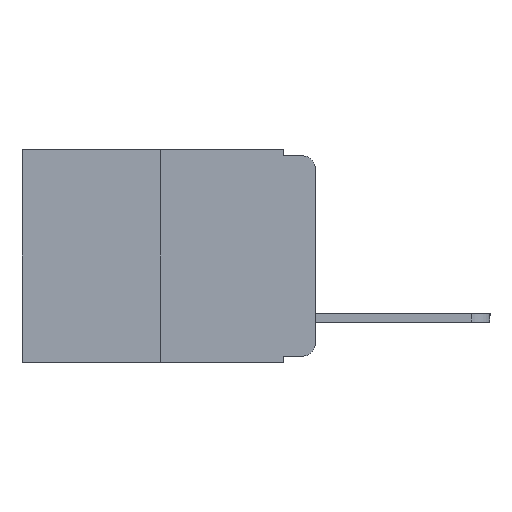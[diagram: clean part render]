
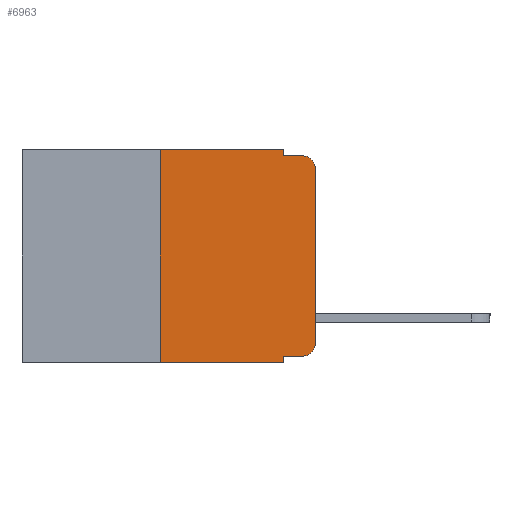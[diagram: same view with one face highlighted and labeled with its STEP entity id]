
A CAD part, left-side view. The second image highlights one B-rep face of the part: STEP entity #6963.
In plain terms, the highlighted planar face has unit normal (-1, 0, 0).
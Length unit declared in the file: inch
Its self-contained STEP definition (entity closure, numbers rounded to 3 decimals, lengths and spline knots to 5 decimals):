
#911 = EDGE_LOOP ( 'NONE', ( #9124, #13321, #1147, #14265, #2266, #7327, #11644, #19059, #3813, #5379 ) ) ;
#1113 = CARTESIAN_POINT ( 'NONE',  ( 0., 0.25, 0. ) ) ;
#1147 = ORIENTED_EDGE ( 'NONE', *, *, #12246, .F. ) ;
#1267 = VECTOR ( 'NONE', #9190, 39.37008 ) ;
#1450 = PLANE ( 'NONE',  #16482 ) ;
#1509 = LINE ( 'NONE', #15160, #9963 ) ;
#1570 = LINE ( 'NONE', #17102, #10512 ) ;
#1821 = LINE ( 'NONE', #10811, #1267 ) ;
#1976 = DIRECTION ( 'NONE',  ( 0., -1., 0. ) ) ;
#2266 = ORIENTED_EDGE ( 'NONE', *, *, #6597, .F. ) ;
#2434 = VERTEX_POINT ( 'NONE', #3434 ) ;
#2712 = EDGE_CURVE ( 'NONE', #18572, #6453, #1509, .T. ) ;
#2749 = VERTEX_POINT ( 'NONE', #3488 ) ;
#3434 = CARTESIAN_POINT ( 'NONE',  ( 0., 0.051, 0. ) ) ;
#3452 = CARTESIAN_POINT ( 'NONE',  ( 0., 0.02, -0.03 ) ) ;
#3488 = CARTESIAN_POINT ( 'NONE',  ( 0., 0.051, -0.333 ) ) ;
#3782 = CARTESIAN_POINT ( 'NONE',  ( 0., 0., 0. ) ) ;
#3813 = ORIENTED_EDGE ( 'NONE', *, *, #15939, .T. ) ;
#3891 = VECTOR ( 'NONE', #7040, 39.37008 ) ;
#3948 = CIRCLE ( 'NONE', #7105, 0.02 ) ;
#4515 = VERTEX_POINT ( 'NONE', #17862 ) ;
#4842 = DIRECTION ( 'NONE',  ( 0., 0., 1. ) ) ;
#5079 = DIRECTION ( 'NONE',  ( 0., 0., -1. ) ) ;
#5379 = ORIENTED_EDGE ( 'NONE', *, *, #11825, .T. ) ;
#5428 = VERTEX_POINT ( 'NONE', #12274 ) ;
#5449 = DIRECTION ( 'NONE',  ( 0., 0., 1. ) ) ;
#5590 = EDGE_CURVE ( 'NONE', #2434, #11676, #1570, .T. ) ;
#5678 = CARTESIAN_POINT ( 'NONE',  ( 0., 0.051, 0. ) ) ;
#5838 = DIRECTION ( 'NONE',  ( -1., 0., 0. ) ) ;
#6208 = VERTEX_POINT ( 'NONE', #19092 ) ;
#6453 = VERTEX_POINT ( 'NONE', #15829 ) ;
#6570 = CARTESIAN_POINT ( 'NONE',  ( 0., 0.051, -0.333 ) ) ;
#6597 = EDGE_CURVE ( 'NONE', #18201, #2434, #8452, .T. ) ;
#6631 = VERTEX_POINT ( 'NONE', #13455 ) ;
#6963 = ADVANCED_FACE ( 'NONE', ( #17617 ), #1450, .F. ) ;
#7040 = DIRECTION ( 'NONE',  ( 0., -1., 0. ) ) ;
#7105 = AXIS2_PLACEMENT_3D ( 'NONE', #15304, #5838, #16618 ) ;
#7327 = ORIENTED_EDGE ( 'NONE', *, *, #16709, .F. ) ;
#7417 = VECTOR ( 'NONE', #5449, 39.37008 ) ;
#8452 = LINE ( 'NONE', #16167, #3891 ) ;
#9124 = ORIENTED_EDGE ( 'NONE', *, *, #18750, .T. ) ;
#9190 = DIRECTION ( 'NONE',  ( 0., -1., 0. ) ) ;
#9215 = VECTOR ( 'NONE', #4842, 39.37008 ) ;
#9225 = LINE ( 'NONE', #5678, #16617 ) ;
#9953 = DIRECTION ( 'NONE',  ( 0., 0., -1. ) ) ;
#9963 = VECTOR ( 'NONE', #1976, 39.37008 ) ;
#10512 = VECTOR ( 'NONE', #17773, 39.37008 ) ;
#10747 = CIRCLE ( 'NONE', #11778, 0.02 ) ;
#10811 = CARTESIAN_POINT ( 'NONE',  ( 0., 0.051, -0.01 ) ) ;
#11644 = ORIENTED_EDGE ( 'NONE', *, *, #2712, .T. ) ;
#11676 = VERTEX_POINT ( 'NONE', #16132 ) ;
#11778 = AXIS2_PLACEMENT_3D ( 'NONE', #3452, #14719, #5079 ) ;
#11825 = EDGE_CURVE ( 'NONE', #5428, #6631, #3948, .T. ) ;
#12236 = LINE ( 'NONE', #6570, #19155 ) ;
#12246 = EDGE_CURVE ( 'NONE', #11676, #6208, #1821, .T. ) ;
#12274 = CARTESIAN_POINT ( 'NONE',  ( 0., 0.02, -0.333 ) ) ;
#13050 = CARTESIAN_POINT ( 'NONE',  ( 0., 0.25, 0. ) ) ;
#13071 = DIRECTION ( 'NONE',  ( 0., -1., 0. ) ) ;
#13321 = ORIENTED_EDGE ( 'NONE', *, *, #16077, .T. ) ;
#13455 = CARTESIAN_POINT ( 'NONE',  ( 0., 0., -0.313 ) ) ;
#14265 = ORIENTED_EDGE ( 'NONE', *, *, #5590, .F. ) ;
#14719 = DIRECTION ( 'NONE',  ( -1., 0., 0. ) ) ;
#15160 = CARTESIAN_POINT ( 'NONE',  ( 0., 0.473, -0.343 ) ) ;
#15304 = CARTESIAN_POINT ( 'NONE',  ( 0., 0.02, -0.313 ) ) ;
#15829 = CARTESIAN_POINT ( 'NONE',  ( 0., 0.051, -0.343 ) ) ;
#15939 = EDGE_CURVE ( 'NONE', #2749, #5428, #12236, .T. ) ;
#16077 = EDGE_CURVE ( 'NONE', #4515, #6208, #10747, .T. ) ;
#16132 = CARTESIAN_POINT ( 'NONE',  ( 0., 0.051, -0.01 ) ) ;
#16167 = CARTESIAN_POINT ( 'NONE',  ( 0., 0.473, 0. ) ) ;
#16482 = AXIS2_PLACEMENT_3D ( 'NONE', #19817, #18536, #9953 ) ;
#16558 = DIRECTION ( 'NONE',  ( 0., 0., -1. ) ) ;
#16617 = VECTOR ( 'NONE', #16558, 39.37008 ) ;
#16618 = DIRECTION ( 'NONE',  ( 0., 0., -1. ) ) ;
#16709 = EDGE_CURVE ( 'NONE', #18572, #18201, #17017, .T. ) ;
#17017 = LINE ( 'NONE', #13050, #9215 ) ;
#17102 = CARTESIAN_POINT ( 'NONE',  ( 0., 0.051, 0. ) ) ;
#17377 = CARTESIAN_POINT ( 'NONE',  ( 0., 0.25, -0.343 ) ) ;
#17617 = FACE_OUTER_BOUND ( 'NONE', #911, .T. ) ;
#17773 = DIRECTION ( 'NONE',  ( 0., 0., -1. ) ) ;
#17862 = CARTESIAN_POINT ( 'NONE',  ( 0., 0., -0.03 ) ) ;
#18201 = VERTEX_POINT ( 'NONE', #1113 ) ;
#18536 = DIRECTION ( 'NONE',  ( 1., 0., 0. ) ) ;
#18572 = VERTEX_POINT ( 'NONE', #17377 ) ;
#18750 = EDGE_CURVE ( 'NONE', #6631, #4515, #19144, .T. ) ;
#18852 = EDGE_CURVE ( 'NONE', #2749, #6453, #9225, .T. ) ;
#19059 = ORIENTED_EDGE ( 'NONE', *, *, #18852, .F. ) ;
#19092 = CARTESIAN_POINT ( 'NONE',  ( 0., 0.02, -0.01 ) ) ;
#19144 = LINE ( 'NONE', #3782, #7417 ) ;
#19155 = VECTOR ( 'NONE', #13071, 39.37008 ) ;
#19817 = CARTESIAN_POINT ( 'NONE',  ( 0., 0.473, 0. ) ) ;
